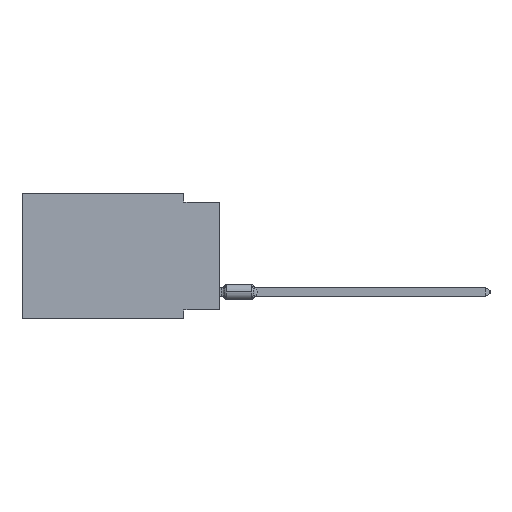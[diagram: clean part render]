
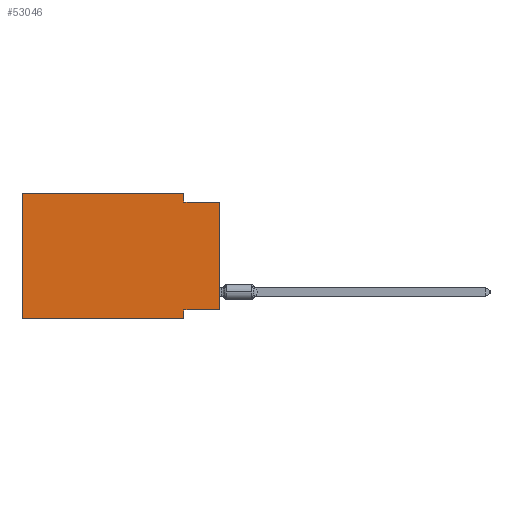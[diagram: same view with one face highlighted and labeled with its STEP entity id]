
A CAD part, left-side view. The second image highlights one B-rep face of the part: STEP entity #53046.
In plain terms, the highlighted planar face has unit normal (-1, 0, 0).
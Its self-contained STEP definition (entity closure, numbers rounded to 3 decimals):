
#1811 = DIRECTION ( 'NONE',  ( 0., 0., -1. ) ) ;
#2285 = LINE ( 'NONE', #54070, #10260 ) ;
#4318 = CARTESIAN_POINT ( 'NONE',  ( 0., 0., -8.255 ) ) ;
#4618 = EDGE_CURVE ( 'NONE', #51885, #26559, #13931, .T. ) ;
#8764 = VERTEX_POINT ( 'NONE', #12311 ) ;
#10260 = VECTOR ( 'NONE', #1811, 1000. ) ;
#12311 = CARTESIAN_POINT ( 'NONE',  ( 0., 2.54, -8.255 ) ) ;
#13082 = VECTOR ( 'NONE', #30160, 1000. ) ;
#13931 = LINE ( 'NONE', #72086, #64785 ) ;
#14607 = CARTESIAN_POINT ( 'NONE',  ( 0., 2.54, -8.89 ) ) ;
#17019 = ORIENTED_EDGE ( 'NONE', *, *, #23765, .F. ) ;
#19776 = EDGE_CURVE ( 'NONE', #68322, #44061, #21956, .T. ) ;
#20142 = LINE ( 'NONE', #78765, #43824 ) ;
#21956 = LINE ( 'NONE', #88873, #89270 ) ;
#22258 = DIRECTION ( 'NONE',  ( 0., -1., 0. ) ) ;
#23765 = EDGE_CURVE ( 'NONE', #8764, #44061, #2285, .T. ) ;
#26559 = VERTEX_POINT ( 'NONE', #64750 ) ;
#29825 = CARTESIAN_POINT ( 'NONE',  ( 0., 13.97, -8.89 ) ) ;
#29837 = EDGE_CURVE ( 'NONE', #80611, #26559, #20142, .T. ) ;
#30160 = DIRECTION ( 'NONE',  ( 0., 0., -1. ) ) ;
#31989 = CARTESIAN_POINT ( 'NONE',  ( 0., 13.97, 0. ) ) ;
#34462 = EDGE_CURVE ( 'NONE', #68322, #89397, #41263, .T. ) ;
#34903 = CARTESIAN_POINT ( 'NONE',  ( 0., 13.97, 0. ) ) ;
#37396 = LINE ( 'NONE', #53035, #86763 ) ;
#38217 = LINE ( 'NONE', #90469, #56448 ) ;
#40615 = VECTOR ( 'NONE', #85232, 1000. ) ;
#41263 = LINE ( 'NONE', #34903, #40615 ) ;
#41445 = ORIENTED_EDGE ( 'NONE', *, *, #4618, .F. ) ;
#43824 = VECTOR ( 'NONE', #55840, 1000. ) ;
#44061 = VERTEX_POINT ( 'NONE', #14607 ) ;
#47159 = PLANE ( 'NONE',  #85193 ) ;
#50583 = DIRECTION ( 'NONE',  ( 0., -1., 0. ) ) ;
#51885 = VERTEX_POINT ( 'NONE', #78840 ) ;
#53035 = CARTESIAN_POINT ( 'NONE',  ( 0., 13.97, 0. ) ) ;
#53046 = ADVANCED_FACE ( 'NONE', ( #92046 ), #47159, .F. ) ;
#53377 = DIRECTION ( 'NONE',  ( 0., 1., 0. ) ) ;
#54070 = CARTESIAN_POINT ( 'NONE',  ( 0., 2.54, -8.89 ) ) ;
#55840 = DIRECTION ( 'NONE',  ( 0., 0., 1. ) ) ;
#56026 = ORIENTED_EDGE ( 'NONE', *, *, #72758, .F. ) ;
#56448 = VECTOR ( 'NONE', #53377, 1000. ) ;
#57560 = ORIENTED_EDGE ( 'NONE', *, *, #19776, .T. ) ;
#61801 = DIRECTION ( 'NONE',  ( 0., 0., -1. ) ) ;
#63974 = EDGE_CURVE ( 'NONE', #89397, #70710, #37396, .T. ) ;
#64750 = CARTESIAN_POINT ( 'NONE',  ( 0., 0., -0.635 ) ) ;
#64785 = VECTOR ( 'NONE', #50583, 1000. ) ;
#68322 = VERTEX_POINT ( 'NONE', #29825 ) ;
#70710 = VERTEX_POINT ( 'NONE', #81928 ) ;
#71603 = EDGE_CURVE ( 'NONE', #80611, #8764, #38217, .T. ) ;
#72086 = CARTESIAN_POINT ( 'NONE',  ( 0., 0., -0.635 ) ) ;
#72758 = EDGE_CURVE ( 'NONE', #70710, #51885, #81930, .T. ) ;
#74615 = CARTESIAN_POINT ( 'NONE',  ( 0., 2.54, 0. ) ) ;
#78672 = ORIENTED_EDGE ( 'NONE', *, *, #34462, .F. ) ;
#78765 = CARTESIAN_POINT ( 'NONE',  ( 0., 0., 0. ) ) ;
#78840 = CARTESIAN_POINT ( 'NONE',  ( 0., 2.54, -0.635 ) ) ;
#79744 = ORIENTED_EDGE ( 'NONE', *, *, #29837, .T. ) ;
#80336 = ORIENTED_EDGE ( 'NONE', *, *, #71603, .F. ) ;
#80611 = VERTEX_POINT ( 'NONE', #4318 ) ;
#81928 = CARTESIAN_POINT ( 'NONE',  ( 0., 2.54, 0. ) ) ;
#81930 = LINE ( 'NONE', #74615, #13082 ) ;
#83293 = CARTESIAN_POINT ( 'NONE',  ( 0., 13.97, 0. ) ) ;
#85193 = AXIS2_PLACEMENT_3D ( 'NONE', #31989, #91582, #61801 ) ;
#85232 = DIRECTION ( 'NONE',  ( 0., 0., 1. ) ) ;
#86763 = VECTOR ( 'NONE', #22258, 1000. ) ;
#87191 = ORIENTED_EDGE ( 'NONE', *, *, #63974, .F. ) ;
#88873 = CARTESIAN_POINT ( 'NONE',  ( 0., 13.97, -8.89 ) ) ;
#89270 = VECTOR ( 'NONE', #96186, 1000. ) ;
#89397 = VERTEX_POINT ( 'NONE', #83293 ) ;
#89535 = EDGE_LOOP ( 'NONE', ( #79744, #41445, #56026, #87191, #78672, #57560, #17019, #80336 ) ) ;
#90469 = CARTESIAN_POINT ( 'NONE',  ( 0., 0., -8.255 ) ) ;
#91582 = DIRECTION ( 'NONE',  ( 1., 0., 0. ) ) ;
#92046 = FACE_OUTER_BOUND ( 'NONE', #89535, .T. ) ;
#96186 = DIRECTION ( 'NONE',  ( 0., -1., 0. ) ) ;
